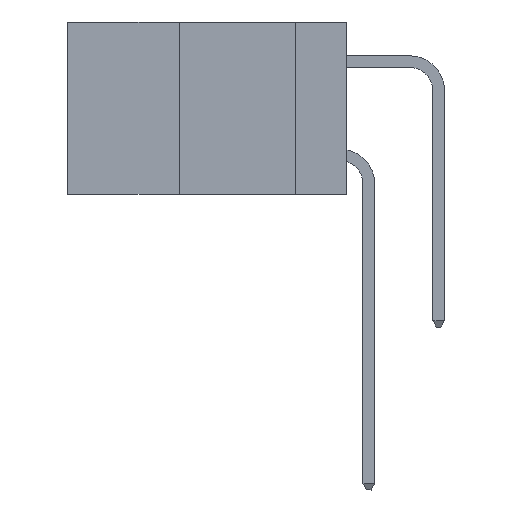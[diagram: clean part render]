
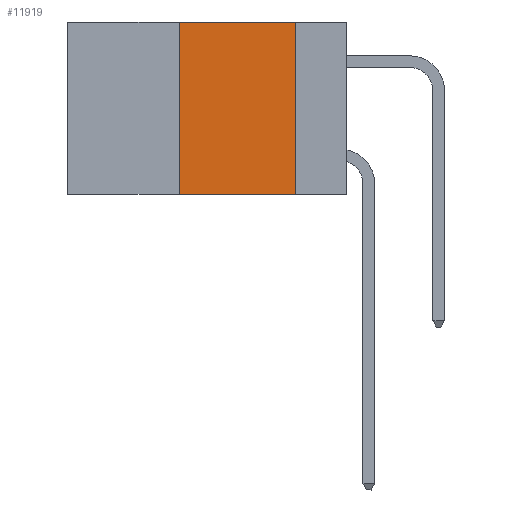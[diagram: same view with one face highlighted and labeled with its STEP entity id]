
A CAD part, left-side view. The second image highlights one B-rep face of the part: STEP entity #11919.
In plain terms, the highlighted planar face has unit normal (-1, 0, 0).
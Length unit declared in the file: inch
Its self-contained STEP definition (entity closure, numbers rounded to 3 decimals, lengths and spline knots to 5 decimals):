
#38 = EDGE_CURVE ( 'NONE', #7909, #1092, #5037, .T. ) ;
#89 = CARTESIAN_POINT ( 'NONE',  ( 0., 0.36, 0. ) ) ;
#500 = EDGE_CURVE ( 'NONE', #1834, #2831, #1002, .T. ) ;
#853 = VECTOR ( 'NONE', #4056, 39.37008 ) ;
#1002 = LINE ( 'NONE', #5122, #853 ) ;
#1092 = VERTEX_POINT ( 'NONE', #3395 ) ;
#1834 = VERTEX_POINT ( 'NONE', #1913 ) ;
#1863 = ORIENTED_EDGE ( 'NONE', *, *, #2250, .F. ) ;
#1913 = CARTESIAN_POINT ( 'NONE',  ( 0., 0.36, 0. ) ) ;
#2081 = VECTOR ( 'NONE', #10050, 39.37008 ) ;
#2250 = EDGE_CURVE ( 'NONE', #7909, #1834, #4991, .T. ) ;
#2831 = VERTEX_POINT ( 'NONE', #5808 ) ;
#2910 = CARTESIAN_POINT ( 'NONE',  ( 0., 0.6, -0.37 ) ) ;
#3395 = CARTESIAN_POINT ( 'NONE',  ( 0., 0.11, -0.37 ) ) ;
#4056 = DIRECTION ( 'NONE',  ( 0., -1., 0. ) ) ;
#4991 = LINE ( 'NONE', #89, #12721 ) ;
#5037 = LINE ( 'NONE', #2910, #2081 ) ;
#5122 = CARTESIAN_POINT ( 'NONE',  ( 0., 0.6, 0. ) ) ;
#5537 = AXIS2_PLACEMENT_3D ( 'NONE', #8731, #11904, #12764 ) ;
#5808 = CARTESIAN_POINT ( 'NONE',  ( 0., 0.11, 0. ) ) ;
#5822 = PLANE ( 'NONE',  #5537 ) ;
#5911 = ORIENTED_EDGE ( 'NONE', *, *, #38, .T. ) ;
#6802 = FACE_OUTER_BOUND ( 'NONE', #11114, .T. ) ;
#6829 = ORIENTED_EDGE ( 'NONE', *, *, #500, .F. ) ;
#7158 = EDGE_CURVE ( 'NONE', #2831, #1092, #11000, .T. ) ;
#7909 = VERTEX_POINT ( 'NONE', #10939 ) ;
#7937 = CARTESIAN_POINT ( 'NONE',  ( 0., 0.11, 0. ) ) ;
#8146 = DIRECTION ( 'NONE',  ( 0., 0., 1. ) ) ;
#8402 = VECTOR ( 'NONE', #11982, 39.37008 ) ;
#8731 = CARTESIAN_POINT ( 'NONE',  ( 0., 0.6, 0. ) ) ;
#8966 = ORIENTED_EDGE ( 'NONE', *, *, #7158, .F. ) ;
#10050 = DIRECTION ( 'NONE',  ( 0., -1., 0. ) ) ;
#10939 = CARTESIAN_POINT ( 'NONE',  ( 0., 0.36, -0.37 ) ) ;
#11000 = LINE ( 'NONE', #7937, #8402 ) ;
#11114 = EDGE_LOOP ( 'NONE', ( #8966, #6829, #1863, #5911 ) ) ;
#11904 = DIRECTION ( 'NONE',  ( 1., 0., 0. ) ) ;
#11919 = ADVANCED_FACE ( 'NONE', ( #6802 ), #5822, .F. ) ;
#11982 = DIRECTION ( 'NONE',  ( 0., 0., -1. ) ) ;
#12721 = VECTOR ( 'NONE', #8146, 39.37008 ) ;
#12764 = DIRECTION ( 'NONE',  ( 0., 0., -1. ) ) ;
